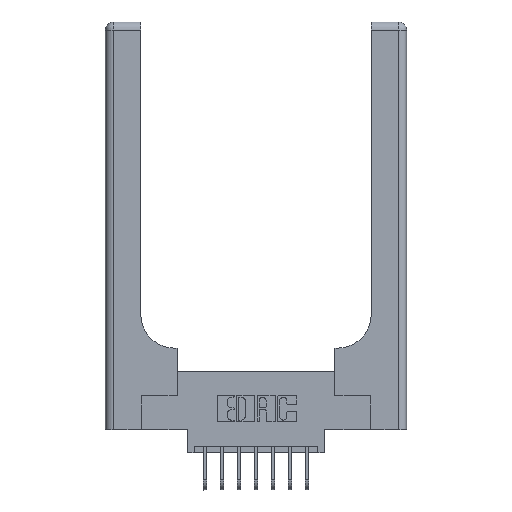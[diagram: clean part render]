
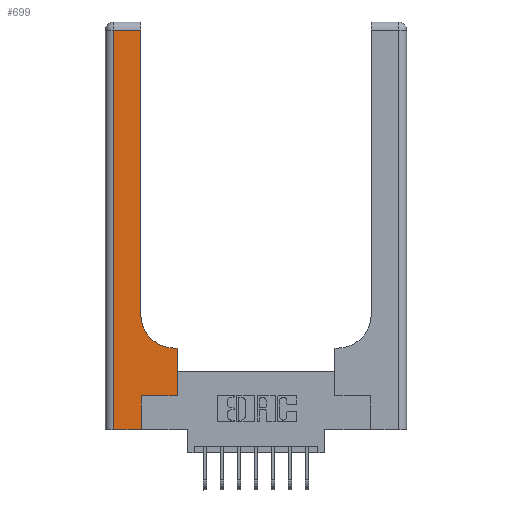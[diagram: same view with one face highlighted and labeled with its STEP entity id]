
A CAD part, top view. The second image highlights one B-rep face of the part: STEP entity #699.
In plain terms, the highlighted planar face has unit normal (0, 0, 1).
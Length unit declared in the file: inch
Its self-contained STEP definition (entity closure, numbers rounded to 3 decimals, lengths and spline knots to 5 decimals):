
#100 = ORIENTED_EDGE ( 'NONE', *, *, #3620, .T. ) ;
#221 = CARTESIAN_POINT ( 'NONE',  ( 0.26, 0.6, 0.37 ) ) ;
#556 = CARTESIAN_POINT ( 'NONE',  ( 0.528, 0.6, 0.37 ) ) ;
#699 = ADVANCED_FACE ( 'NONE', ( #1268 ), #7456, .F. ) ;
#954 = DIRECTION ( 'NONE',  ( 1., 0., 0. ) ) ;
#1071 = VERTEX_POINT ( 'NONE', #1474 ) ;
#1142 = VECTOR ( 'NONE', #8581, 39.37008 ) ;
#1238 = CARTESIAN_POINT ( 'NONE',  ( 0.26, 2.94, 0.37 ) ) ;
#1268 = FACE_OUTER_BOUND ( 'NONE', #10088, .T. ) ;
#1321 = VECTOR ( 'NONE', #14370, 39.37008 ) ;
#1474 = CARTESIAN_POINT ( 'NONE',  ( 0.06, 2.94, 0.37 ) ) ;
#1480 = VERTEX_POINT ( 'NONE', #10337 ) ;
#1773 = DIRECTION ( 'NONE',  ( -1., 0., 0. ) ) ;
#1822 = CARTESIAN_POINT ( 'NONE',  ( 0.26, 3., 0.37 ) ) ;
#2018 = VECTOR ( 'NONE', #9317, 39.37008 ) ;
#2128 = LINE ( 'NONE', #7739, #13609 ) ;
#3620 = EDGE_CURVE ( 'NONE', #1071, #8000, #2128, .T. ) ;
#3982 = AXIS2_PLACEMENT_3D ( 'NONE', #4181, #11984, #5314 ) ;
#4094 = CARTESIAN_POINT ( 'NONE',  ( 0.528, 0.25, 0.37 ) ) ;
#4181 = CARTESIAN_POINT ( 'NONE',  ( 0.51, 0.85, 0.37 ) ) ;
#4204 = LINE ( 'NONE', #1822, #1142 ) ;
#4243 = ORIENTED_EDGE ( 'NONE', *, *, #6217, .T. ) ;
#4344 = VERTEX_POINT ( 'NONE', #4094 ) ;
#4386 = CARTESIAN_POINT ( 'NONE',  ( 0.265, 0.25, 0.37 ) ) ;
#4911 = LINE ( 'NONE', #10766, #13389 ) ;
#5047 = LINE ( 'NONE', #221, #2018 ) ;
#5314 = DIRECTION ( 'NONE',  ( 1., 0., 0. ) ) ;
#5469 = CARTESIAN_POINT ( 'NONE',  ( 0.528, 0.25, 0.37 ) ) ;
#5548 = DIRECTION ( 'NONE',  ( 0., -1., 0. ) ) ;
#5974 = ORIENTED_EDGE ( 'NONE', *, *, #6035, .T. ) ;
#6010 = EDGE_CURVE ( 'NONE', #8000, #1480, #4911, .T. ) ;
#6035 = EDGE_CURVE ( 'NONE', #11410, #8124, #4204, .T. ) ;
#6217 = EDGE_CURVE ( 'NONE', #1480, #10999, #10322, .T. ) ;
#6247 = CARTESIAN_POINT ( 'NONE',  ( 0., 3., 0.37 ) ) ;
#6710 = ORIENTED_EDGE ( 'NONE', *, *, #6010, .T. ) ;
#7053 = ORIENTED_EDGE ( 'NONE', *, *, #12622, .T. ) ;
#7127 = VERTEX_POINT ( 'NONE', #556 ) ;
#7456 = PLANE ( 'NONE',  #12660 ) ;
#7696 = CARTESIAN_POINT ( 'NONE',  ( 0.26, 0.85, 0.37 ) ) ;
#7739 = CARTESIAN_POINT ( 'NONE',  ( 0.06, 3., 0.37 ) ) ;
#8000 = VERTEX_POINT ( 'NONE', #13314 ) ;
#8124 = VERTEX_POINT ( 'NONE', #1238 ) ;
#8391 = CARTESIAN_POINT ( 'NONE',  ( 0., 2.94, 0.37 ) ) ;
#8581 = DIRECTION ( 'NONE',  ( 0., 1., 0. ) ) ;
#8986 = CARTESIAN_POINT ( 'NONE',  ( 0.51, 0.6, 0.37 ) ) ;
#9229 = VECTOR ( 'NONE', #9583, 39.37008 ) ;
#9317 = DIRECTION ( 'NONE',  ( -1., 0., 0. ) ) ;
#9425 = VERTEX_POINT ( 'NONE', #8986 ) ;
#9583 = DIRECTION ( 'NONE',  ( -1., 0., 0. ) ) ;
#9713 = EDGE_CURVE ( 'NONE', #9425, #11410, #10175, .T. ) ;
#9759 = EDGE_CURVE ( 'NONE', #10999, #4344, #9829, .T. ) ;
#9829 = LINE ( 'NONE', #4386, #12432 ) ;
#9904 = DIRECTION ( 'NONE',  ( 0., 1., 0. ) ) ;
#10083 = LINE ( 'NONE', #5469, #12665 ) ;
#10088 = EDGE_LOOP ( 'NONE', ( #5974, #11883, #100, #6710, #4243, #12403, #10418, #7053, #10933 ) ) ;
#10175 = CIRCLE ( 'NONE', #3982, 0.25 ) ;
#10322 = LINE ( 'NONE', #13332, #1321 ) ;
#10337 = CARTESIAN_POINT ( 'NONE',  ( 0.265, 0., 0.37 ) ) ;
#10418 = ORIENTED_EDGE ( 'NONE', *, *, #13854, .T. ) ;
#10766 = CARTESIAN_POINT ( 'NONE',  ( 0., 0., 0.37 ) ) ;
#10933 = ORIENTED_EDGE ( 'NONE', *, *, #9713, .T. ) ;
#10999 = VERTEX_POINT ( 'NONE', #11411 ) ;
#11410 = VERTEX_POINT ( 'NONE', #7696 ) ;
#11411 = CARTESIAN_POINT ( 'NONE',  ( 0.265, 0.25, 0.37 ) ) ;
#11799 = DIRECTION ( 'NONE',  ( 0., 0., -1. ) ) ;
#11883 = ORIENTED_EDGE ( 'NONE', *, *, #13228, .T. ) ;
#11984 = DIRECTION ( 'NONE',  ( 0., 0., -1. ) ) ;
#12194 = LINE ( 'NONE', #8391, #9229 ) ;
#12403 = ORIENTED_EDGE ( 'NONE', *, *, #9759, .T. ) ;
#12432 = VECTOR ( 'NONE', #954, 39.37008 ) ;
#12622 = EDGE_CURVE ( 'NONE', #7127, #9425, #5047, .T. ) ;
#12660 = AXIS2_PLACEMENT_3D ( 'NONE', #6247, #11799, #1773 ) ;
#12665 = VECTOR ( 'NONE', #9904, 39.37008 ) ;
#12935 = DIRECTION ( 'NONE',  ( 1., 0., 0. ) ) ;
#13228 = EDGE_CURVE ( 'NONE', #8124, #1071, #12194, .T. ) ;
#13314 = CARTESIAN_POINT ( 'NONE',  ( 0.06, 0., 0.37 ) ) ;
#13332 = CARTESIAN_POINT ( 'NONE',  ( 0.265, 0., 0.37 ) ) ;
#13389 = VECTOR ( 'NONE', #12935, 39.37008 ) ;
#13609 = VECTOR ( 'NONE', #5548, 39.37008 ) ;
#13854 = EDGE_CURVE ( 'NONE', #4344, #7127, #10083, .T. ) ;
#14370 = DIRECTION ( 'NONE',  ( 0., 1., 0. ) ) ;
